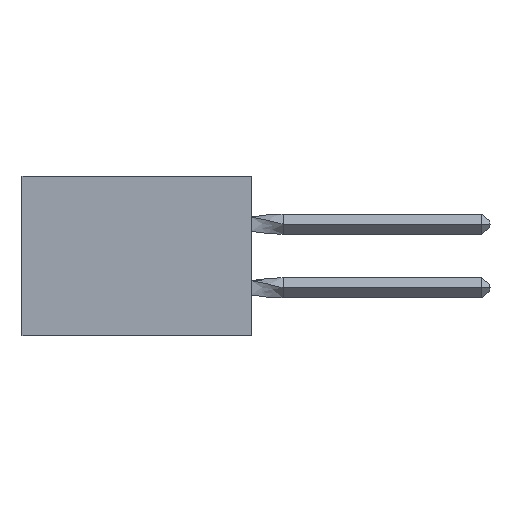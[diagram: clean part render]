
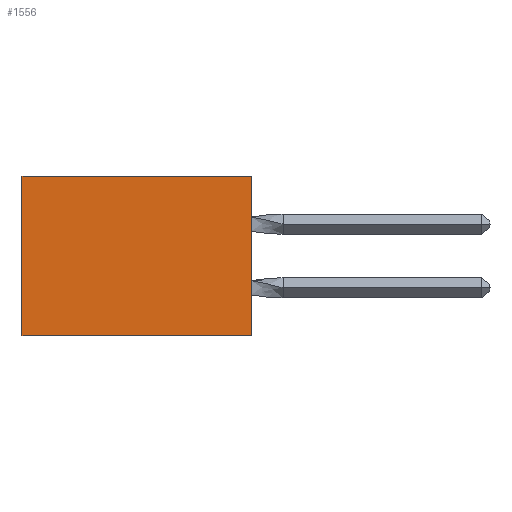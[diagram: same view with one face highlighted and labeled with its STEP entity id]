
A CAD part, left-side view. The second image highlights one B-rep face of the part: STEP entity #1556.
In plain terms, the highlighted planar face has unit normal (-1, 0, 0).
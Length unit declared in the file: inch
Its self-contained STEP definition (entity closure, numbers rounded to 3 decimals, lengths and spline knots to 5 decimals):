
#721 = LINE ( 'NONE', #19198, #12139 ) ;
#916 = CARTESIAN_POINT ( 'NONE',  ( 0.305, 0., -0.5 ) ) ;
#1556 = ADVANCED_FACE ( 'NONE', ( #14032 ), #4147, .F. ) ;
#2495 = LINE ( 'NONE', #2544, #11376 ) ;
#2544 = CARTESIAN_POINT ( 'NONE',  ( 0.305, 0., -0.5 ) ) ;
#3479 = ORIENTED_EDGE ( 'NONE', *, *, #20728, .F. ) ;
#3533 = LINE ( 'NONE', #12680, #12170 ) ;
#4147 = PLANE ( 'NONE',  #14162 ) ;
#4265 = EDGE_CURVE ( 'NONE', #11059, #19778, #2495, .T. ) ;
#4968 = EDGE_CURVE ( 'NONE', #15017, #13810, #721, .T. ) ;
#5589 = VECTOR ( 'NONE', #17069, 39.37008 ) ;
#5813 = DIRECTION ( 'NONE',  ( 0., 0., -1. ) ) ;
#7122 = CARTESIAN_POINT ( 'NONE',  ( 0.305, 0., -0.5 ) ) ;
#7962 = DIRECTION ( 'NONE',  ( 0., 1., 0. ) ) ;
#8189 = ORIENTED_EDGE ( 'NONE', *, *, #4968, .T. ) ;
#10378 = CARTESIAN_POINT ( 'NONE',  ( 0.305, 0., -0.5 ) ) ;
#10681 = EDGE_CURVE ( 'NONE', #11059, #15017, #3533, .T. ) ;
#11059 = VERTEX_POINT ( 'NONE', #20409 ) ;
#11376 = VECTOR ( 'NONE', #5813, 39.37008 ) ;
#11905 = CARTESIAN_POINT ( 'NONE',  ( 0.305, 0.72, -0.5 ) ) ;
#12139 = VECTOR ( 'NONE', #19052, 39.37008 ) ;
#12170 = VECTOR ( 'NONE', #7962, 39.37008 ) ;
#12680 = CARTESIAN_POINT ( 'NONE',  ( 0.305, 0., 0. ) ) ;
#13810 = VERTEX_POINT ( 'NONE', #11905 ) ;
#14032 = FACE_OUTER_BOUND ( 'NONE', #15358, .T. ) ;
#14162 = AXIS2_PLACEMENT_3D ( 'NONE', #916, #18566, #15450 ) ;
#15017 = VERTEX_POINT ( 'NONE', #15275 ) ;
#15275 = CARTESIAN_POINT ( 'NONE',  ( 0.305, 0.72, 0. ) ) ;
#15358 = EDGE_LOOP ( 'NONE', ( #8189, #3479, #20325, #17858 ) ) ;
#15450 = DIRECTION ( 'NONE',  ( 0., 0., -1. ) ) ;
#16987 = LINE ( 'NONE', #10378, #5589 ) ;
#17069 = DIRECTION ( 'NONE',  ( 0., 1., 0. ) ) ;
#17858 = ORIENTED_EDGE ( 'NONE', *, *, #10681, .T. ) ;
#18566 = DIRECTION ( 'NONE',  ( 1., 0., 0. ) ) ;
#19052 = DIRECTION ( 'NONE',  ( 0., 0., -1. ) ) ;
#19198 = CARTESIAN_POINT ( 'NONE',  ( 0.305, 0.72, -0.5 ) ) ;
#19778 = VERTEX_POINT ( 'NONE', #7122 ) ;
#20325 = ORIENTED_EDGE ( 'NONE', *, *, #4265, .F. ) ;
#20409 = CARTESIAN_POINT ( 'NONE',  ( 0.305, 0., 0. ) ) ;
#20728 = EDGE_CURVE ( 'NONE', #19778, #13810, #16987, .T. ) ;
